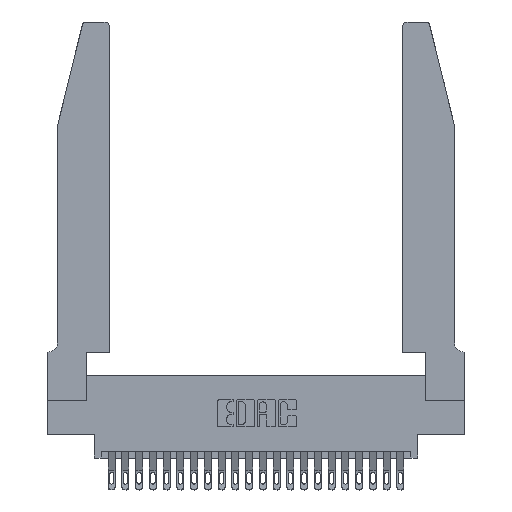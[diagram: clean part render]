
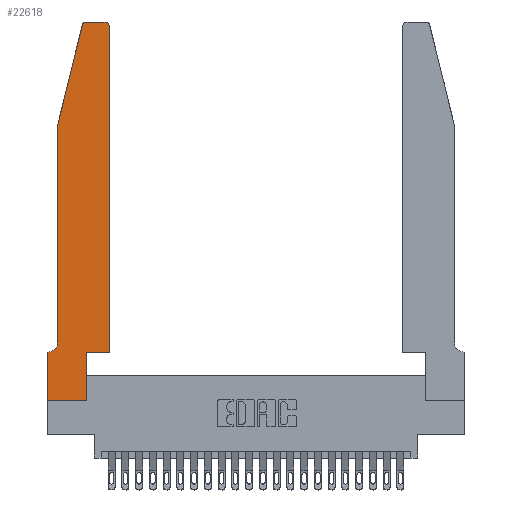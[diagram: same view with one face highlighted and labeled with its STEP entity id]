
A CAD part, top view. The second image highlights one B-rep face of the part: STEP entity #22618.
In plain terms, the highlighted planar face has unit normal (0, 0, 1).
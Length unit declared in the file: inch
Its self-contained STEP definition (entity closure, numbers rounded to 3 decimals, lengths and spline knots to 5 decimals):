
#107 = ORIENTED_EDGE ( 'NONE', *, *, #24803, .T. ) ;
#164 = CIRCLE ( 'NONE', #9795, 0.03 ) ;
#391 = LINE ( 'NONE', #3325, #10279 ) ;
#551 = CARTESIAN_POINT ( 'NONE',  ( 0.25487, 2.72718, 0.37 ) ) ;
#804 = ORIENTED_EDGE ( 'NONE', *, *, #16401, .T. ) ;
#922 = LINE ( 'NONE', #11304, #20408 ) ;
#1084 = PLANE ( 'NONE',  #14046 ) ;
#1165 = EDGE_LOOP ( 'NONE', ( #18208, #16644, #804, #11325, #18204, #107, #4728, #12675, #3962, #23590, #13339, #13201 ) ) ;
#1175 = DIRECTION ( 'NONE',  ( 0., 0., 1. ) ) ;
#1311 = EDGE_CURVE ( 'NONE', #3235, #9612, #13876, .T. ) ;
#2501 = VERTEX_POINT ( 'NONE', #14879 ) ;
#2914 = VECTOR ( 'NONE', #13070, 39.37008 ) ;
#3235 = VERTEX_POINT ( 'NONE', #23793 ) ;
#3325 = CARTESIAN_POINT ( 'NONE',  ( 0.0755, 0.35, 0.37 ) ) ;
#3777 = VERTEX_POINT ( 'NONE', #21588 ) ;
#3962 = ORIENTED_EDGE ( 'NONE', *, *, #21202, .T. ) ;
#4728 = ORIENTED_EDGE ( 'NONE', *, *, #12658, .T. ) ;
#4887 = DIRECTION ( 'NONE',  ( 0., 0., 1. ) ) ;
#5098 = VECTOR ( 'NONE', #17919, 39.37008 ) ;
#5300 = DIRECTION ( 'NONE',  ( -1., 0., 0. ) ) ;
#5414 = DIRECTION ( 'NONE',  ( -1., 0., 0. ) ) ;
#5455 = CIRCLE ( 'NONE', #23386, 0.07 ) ;
#6264 = EDGE_CURVE ( 'NONE', #12129, #24423, #922, .T. ) ;
#6363 = CARTESIAN_POINT ( 'NONE',  ( 0.2865, 0.35, 0.37 ) ) ;
#7054 = CARTESIAN_POINT ( 'NONE',  ( 0.0055, 0.35, 0.37 ) ) ;
#7061 = EDGE_CURVE ( 'NONE', #24366, #3235, #13782, .T. ) ;
#8534 = VERTEX_POINT ( 'NONE', #10554 ) ;
#8554 = CARTESIAN_POINT ( 'NONE',  ( 0.0055, 0.42, 0.37 ) ) ;
#8785 = CIRCLE ( 'NONE', #14369, 0.03 ) ;
#9374 = LINE ( 'NONE', #12536, #24731 ) ;
#9407 = VERTEX_POINT ( 'NONE', #18745 ) ;
#9612 = VERTEX_POINT ( 'NONE', #17916 ) ;
#9795 = AXIS2_PLACEMENT_3D ( 'NONE', #22786, #11277, #24683 ) ;
#10279 = VECTOR ( 'NONE', #5300, 39.37008 ) ;
#10446 = EDGE_CURVE ( 'NONE', #9612, #12129, #8785, .T. ) ;
#10507 = DIRECTION ( 'NONE',  ( -1., 0., 0. ) ) ;
#10554 = CARTESIAN_POINT ( 'NONE',  ( 0.0755, 2., 0.37 ) ) ;
#10892 = EDGE_CURVE ( 'NONE', #8534, #2501, #9374, .T. ) ;
#11277 = DIRECTION ( 'NONE',  ( 0., 0., 1. ) ) ;
#11304 = CARTESIAN_POINT ( 'NONE',  ( 0.2605, 2.75, 0.37 ) ) ;
#11325 = ORIENTED_EDGE ( 'NONE', *, *, #10892, .T. ) ;
#11920 = FACE_OUTER_BOUND ( 'NONE', #1165, .T. ) ;
#12129 = VERTEX_POINT ( 'NONE', #24024 ) ;
#12536 = CARTESIAN_POINT ( 'NONE',  ( 0.0755, 2., 0.37 ) ) ;
#12658 = EDGE_CURVE ( 'NONE', #13573, #3777, #13274, .T. ) ;
#12675 = ORIENTED_EDGE ( 'NONE', *, *, #12880, .T. ) ;
#12717 = DIRECTION ( 'NONE',  ( -0.239, -0.971, 0. ) ) ;
#12880 = EDGE_CURVE ( 'NONE', #3777, #9407, #13566, .T. ) ;
#13070 = DIRECTION ( 'NONE',  ( 0., -1., 0. ) ) ;
#13201 = ORIENTED_EDGE ( 'NONE', *, *, #10446, .T. ) ;
#13274 = LINE ( 'NONE', #22729, #2914 ) ;
#13339 = ORIENTED_EDGE ( 'NONE', *, *, #1311, .T. ) ;
#13566 = LINE ( 'NONE', #15734, #23178 ) ;
#13573 = VERTEX_POINT ( 'NONE', #16302 ) ;
#13782 = LINE ( 'NONE', #17349, #18243 ) ;
#13789 = CARTESIAN_POINT ( 'NONE',  ( 0.2865, 0.35, 0.37 ) ) ;
#13876 = LINE ( 'NONE', #23927, #23490 ) ;
#14046 = AXIS2_PLACEMENT_3D ( 'NONE', #20569, #1175, #14884 ) ;
#14369 = AXIS2_PLACEMENT_3D ( 'NONE', #16492, #4887, #18370 ) ;
#14743 = VECTOR ( 'NONE', #12717, 39.37008 ) ;
#14879 = CARTESIAN_POINT ( 'NONE',  ( 0.0755, 0.42, 0.37 ) ) ;
#14884 = DIRECTION ( 'NONE',  ( 1., 0., 0. ) ) ;
#15734 = CARTESIAN_POINT ( 'NONE',  ( 0., 0., 0.37 ) ) ;
#15802 = CARTESIAN_POINT ( 'NONE',  ( 0.284, 2.75, 0.37 ) ) ;
#16302 = CARTESIAN_POINT ( 'NONE',  ( 0., 0.35, 0.37 ) ) ;
#16401 = EDGE_CURVE ( 'NONE', #22456, #8534, #19810, .T. ) ;
#16492 = CARTESIAN_POINT ( 'NONE',  ( 0.4205, 2.72, 0.37 ) ) ;
#16644 = ORIENTED_EDGE ( 'NONE', *, *, #19149, .T. ) ;
#17349 = CARTESIAN_POINT ( 'NONE',  ( 0.4505, 0.35, 0.37 ) ) ;
#17645 = DIRECTION ( 'NONE',  ( 1., 0., 0. ) ) ;
#17916 = CARTESIAN_POINT ( 'NONE',  ( 0.4505, 2.72, 0.37 ) ) ;
#17919 = DIRECTION ( 'NONE',  ( 0., 1., 0. ) ) ;
#18204 = ORIENTED_EDGE ( 'NONE', *, *, #23626, .T. ) ;
#18208 = ORIENTED_EDGE ( 'NONE', *, *, #6264, .T. ) ;
#18243 = VECTOR ( 'NONE', #19248, 39.37008 ) ;
#18370 = DIRECTION ( 'NONE',  ( 1., 0., 0. ) ) ;
#18745 = CARTESIAN_POINT ( 'NONE',  ( 0.2865, 0., 0.37 ) ) ;
#19149 = EDGE_CURVE ( 'NONE', #24423, #22456, #164, .T. ) ;
#19248 = DIRECTION ( 'NONE',  ( 1., 0., 0. ) ) ;
#19810 = LINE ( 'NONE', #22275, #14743 ) ;
#20228 = VERTEX_POINT ( 'NONE', #7054 ) ;
#20408 = VECTOR ( 'NONE', #5414, 39.37008 ) ;
#20486 = LINE ( 'NONE', #6363, #5098 ) ;
#20569 = CARTESIAN_POINT ( 'NONE',  ( 0., 0.35, 0.37 ) ) ;
#21202 = EDGE_CURVE ( 'NONE', #9407, #24366, #20486, .T. ) ;
#21588 = CARTESIAN_POINT ( 'NONE',  ( 0., 0., 0.37 ) ) ;
#22029 = DIRECTION ( 'NONE',  ( 0., 0., -1. ) ) ;
#22275 = CARTESIAN_POINT ( 'NONE',  ( 0.0755, 2., 0.37 ) ) ;
#22456 = VERTEX_POINT ( 'NONE', #551 ) ;
#22618 = ADVANCED_FACE ( 'NONE', ( #11920 ), #1084, .T. ) ;
#22729 = CARTESIAN_POINT ( 'NONE',  ( 0., 0., 0.37 ) ) ;
#22786 = CARTESIAN_POINT ( 'NONE',  ( 0.284, 2.72, 0.37 ) ) ;
#23178 = VECTOR ( 'NONE', #17645, 39.37008 ) ;
#23386 = AXIS2_PLACEMENT_3D ( 'NONE', #8554, #22029, #10507 ) ;
#23490 = VECTOR ( 'NONE', #24748, 39.37008 ) ;
#23590 = ORIENTED_EDGE ( 'NONE', *, *, #7061, .T. ) ;
#23626 = EDGE_CURVE ( 'NONE', #2501, #20228, #5455, .T. ) ;
#23741 = DIRECTION ( 'NONE',  ( 0., -1., 0. ) ) ;
#23793 = CARTESIAN_POINT ( 'NONE',  ( 0.4505, 0.35, 0.37 ) ) ;
#23927 = CARTESIAN_POINT ( 'NONE',  ( 0.4505, 0.35, 0.37 ) ) ;
#24024 = CARTESIAN_POINT ( 'NONE',  ( 0.4205, 2.75, 0.37 ) ) ;
#24366 = VERTEX_POINT ( 'NONE', #13789 ) ;
#24423 = VERTEX_POINT ( 'NONE', #15802 ) ;
#24683 = DIRECTION ( 'NONE',  ( 1., 0., 0. ) ) ;
#24731 = VECTOR ( 'NONE', #23741, 39.37008 ) ;
#24748 = DIRECTION ( 'NONE',  ( 0., 1., 0. ) ) ;
#24803 = EDGE_CURVE ( 'NONE', #20228, #13573, #391, .T. ) ;
